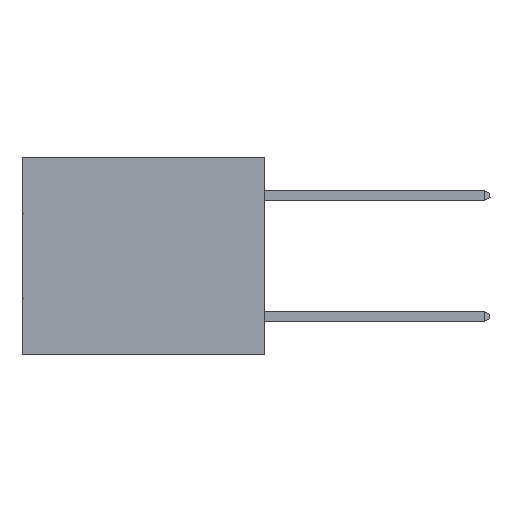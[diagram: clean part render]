
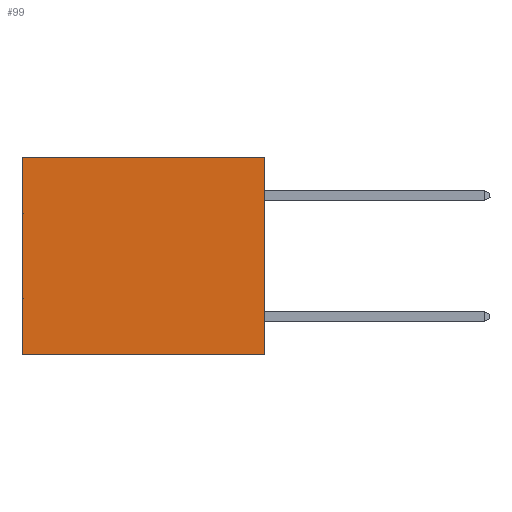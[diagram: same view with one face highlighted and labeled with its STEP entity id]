
A CAD part, left-side view. The second image highlights one B-rep face of the part: STEP entity #99.
In plain terms, the highlighted planar face has unit normal (-1, 0, 0).
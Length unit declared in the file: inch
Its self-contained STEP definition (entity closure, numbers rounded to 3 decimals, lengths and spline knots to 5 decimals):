
#99 = ADVANCED_FACE ( 'NONE', ( #29255 ), #19687, .F. ) ;
#1246 = DIRECTION ( 'NONE',  ( 0., 0., -1. ) ) ;
#1443 = EDGE_CURVE ( 'NONE', #16965, #17087, #24914, .T. ) ;
#1960 = CARTESIAN_POINT ( 'NONE',  ( 0.3165, 0., -0.49 ) ) ;
#2181 = DIRECTION ( 'NONE',  ( 0., 1., 0. ) ) ;
#4363 = LINE ( 'NONE', #23295, #24604 ) ;
#7618 = VECTOR ( 'NONE', #2181, 39.37008 ) ;
#7665 = AXIS2_PLACEMENT_3D ( 'NONE', #25326, #17437, #1246 ) ;
#8668 = CARTESIAN_POINT ( 'NONE',  ( 0.3165, 0., 0. ) ) ;
#13771 = ORIENTED_EDGE ( 'NONE', *, *, #1443, .F. ) ;
#14631 = EDGE_LOOP ( 'NONE', ( #17895, #13771, #30184, #33740 ) ) ;
#16604 = DIRECTION ( 'NONE',  ( 0., 1., 0. ) ) ;
#16965 = VERTEX_POINT ( 'NONE', #29725 ) ;
#17087 = VERTEX_POINT ( 'NONE', #27841 ) ;
#17437 = DIRECTION ( 'NONE',  ( 1., 0., 0. ) ) ;
#17895 = ORIENTED_EDGE ( 'NONE', *, *, #32307, .T. ) ;
#18567 = DIRECTION ( 'NONE',  ( 0., 0., -1. ) ) ;
#19009 = VECTOR ( 'NONE', #16604, 39.37008 ) ;
#19687 = PLANE ( 'NONE',  #7665 ) ;
#21143 = CARTESIAN_POINT ( 'NONE',  ( 0.3165, 0.6, -0.49 ) ) ;
#21160 = VERTEX_POINT ( 'NONE', #22368 ) ;
#21593 = CARTESIAN_POINT ( 'NONE',  ( 0.3165, 0.6, 0. ) ) ;
#21889 = LINE ( 'NONE', #21143, #34580 ) ;
#22368 = CARTESIAN_POINT ( 'NONE',  ( 0.3165, 0., 0. ) ) ;
#22943 = DIRECTION ( 'NONE',  ( 0., 0., -1. ) ) ;
#23295 = CARTESIAN_POINT ( 'NONE',  ( 0.3165, 0., -0.49 ) ) ;
#24502 = EDGE_CURVE ( 'NONE', #21160, #16965, #4363, .T. ) ;
#24604 = VECTOR ( 'NONE', #22943, 39.37008 ) ;
#24914 = LINE ( 'NONE', #1960, #7618 ) ;
#25326 = CARTESIAN_POINT ( 'NONE',  ( 0.3165, 0., -0.49 ) ) ;
#27841 = CARTESIAN_POINT ( 'NONE',  ( 0.3165, 0.6, -0.49 ) ) ;
#29255 = FACE_OUTER_BOUND ( 'NONE', #14631, .T. ) ;
#29525 = LINE ( 'NONE', #8668, #19009 ) ;
#29725 = CARTESIAN_POINT ( 'NONE',  ( 0.3165, 0., -0.49 ) ) ;
#30184 = ORIENTED_EDGE ( 'NONE', *, *, #24502, .F. ) ;
#31948 = EDGE_CURVE ( 'NONE', #21160, #34159, #29525, .T. ) ;
#32307 = EDGE_CURVE ( 'NONE', #34159, #17087, #21889, .T. ) ;
#33740 = ORIENTED_EDGE ( 'NONE', *, *, #31948, .T. ) ;
#34159 = VERTEX_POINT ( 'NONE', #21593 ) ;
#34580 = VECTOR ( 'NONE', #18567, 39.37008 ) ;
